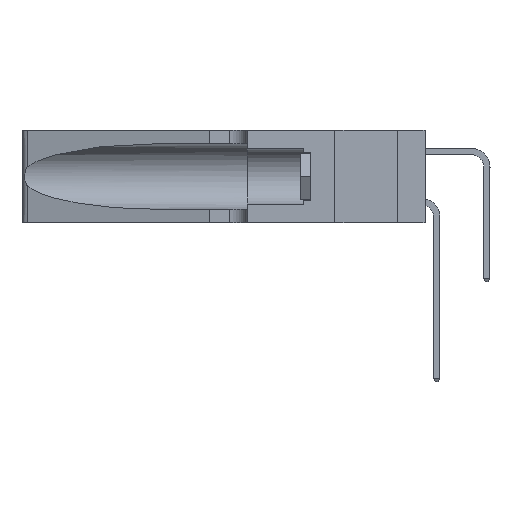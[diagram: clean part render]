
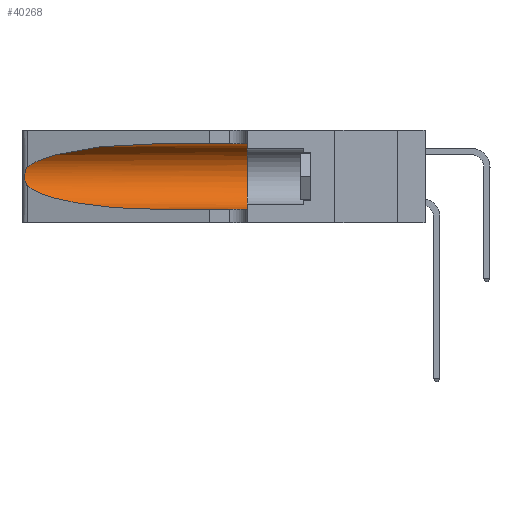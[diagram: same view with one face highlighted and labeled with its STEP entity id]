
A CAD part, left-side view. The second image highlights one B-rep face of the part: STEP entity #40268.
In plain terms, the highlighted cylindrical face has radius 3.308 mm (diameter 6.617 mm), a partial arc.
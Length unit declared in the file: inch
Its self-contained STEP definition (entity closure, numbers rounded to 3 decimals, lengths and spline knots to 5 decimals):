
#661 = B_SPLINE_CURVE_WITH_KNOTS ( 'NONE', 3,
 ( #7640, #23394, #4822, #4966, #5103, #8390, #40996, #11251, #28452, #34728, #28595, #31602, #32160, #907 ),
 .UNSPECIFIED., .F., .F.,
 ( 4, 2, 2, 2, 2, 2, 4 ),
 ( 0., 0.00027, 0.00053, 0.00107, 0.0016, 0.00187, 0.00214 ),
 .UNSPECIFIED. ) ;
#907 = CARTESIAN_POINT ( 'NONE',  ( 0.25487, 1.22718, 0.14631 ) ) ;
#982 = AXIS2_PLACEMENT_3D ( 'NONE', #37125, #40444, #34043 ) ;
#1090 = CARTESIAN_POINT ( 'NONE',  ( 0.25487, 1.22718, 0.22369 ) ) ;
#1676 = CARTESIAN_POINT ( 'NONE',  ( 0.18966, 0.96281, 0.05475 ) ) ;
#1841 = CARTESIAN_POINT ( 'NONE',  ( 0.1305, 1.61858, 0.05475 ) ) ;
#3299 = FACE_OUTER_BOUND ( 'NONE', #30682, .T. ) ;
#3983 = ORIENTED_EDGE ( 'NONE', *, *, #23581, .T. ) ;
#4087 = CARTESIAN_POINT ( 'NONE',  ( 0.1305, 0.35, 0.31525 ) ) ;
#4822 = CARTESIAN_POINT ( 'NONE',  ( 0.25639, 1.23184, 0.21858 ) ) ;
#4966 = CARTESIAN_POINT ( 'NONE',  ( 0.25787, 1.23484, 0.2124 ) ) ;
#5041 = CARTESIAN_POINT ( 'NONE',  ( 0.1305, 1.61858, 0.31525 ) ) ;
#5103 = CARTESIAN_POINT ( 'NONE',  ( 0.25854, 1.2359, 0.20912 ) ) ;
#6863 = DIRECTION ( 'NONE',  ( 0., 1., 0. ) ) ;
#6898 = CARTESIAN_POINT ( 'NONE',  ( 0.1305, 0.72297, 0.31525 ) ) ;
#7305 = CARTESIAN_POINT ( 'NONE',  ( 0.2373, 1.15595, 0.08982 ) ) ;
#7470 = CARTESIAN_POINT ( 'NONE',  ( 0.2373, 1.15595, 0.28018 ) ) ;
#7640 = CARTESIAN_POINT ( 'NONE',  ( 0.25487, 1.22718, 0.22369 ) ) ;
#7692 =( BOUNDED_CURVE ( )  B_SPLINE_CURVE ( 3, ( #14309, #7305, #1676, #37330 ),
 .UNSPECIFIED., .F., .F. ) 
 B_SPLINE_CURVE_WITH_KNOTS ( ( 4, 4 ),
 ( 3.44316, 4.71239 ),
 .UNSPECIFIED. ) 
 CURVE ( )  GEOMETRIC_REPRESENTATION_ITEM ( )  RATIONAL_B_SPLINE_CURVE ( ( 1., 0.87, 0.87, 1. ) ) 
 REPRESENTATION_ITEM ( '' )  );
#8259 =( BOUNDED_CURVE ( )  B_SPLINE_CURVE ( 3, ( #36243, #10764, #7470, #1090 ),
 .UNSPECIFIED., .F., .F. ) 
 B_SPLINE_CURVE_WITH_KNOTS ( ( 4, 4 ),
 ( 1.5708, 2.84003 ),
 .UNSPECIFIED. ) 
 CURVE ( )  GEOMETRIC_REPRESENTATION_ITEM ( )  RATIONAL_B_SPLINE_CURVE ( ( 1., 0.87, 0.87, 1. ) ) 
 REPRESENTATION_ITEM ( '' )  );
#8390 = CARTESIAN_POINT ( 'NONE',  ( 0.26018, 1.23835, 0.19895 ) ) ;
#10563 = VECTOR ( 'NONE', #34265, 39.37008 ) ;
#10764 = CARTESIAN_POINT ( 'NONE',  ( 0.18966, 0.96281, 0.31525 ) ) ;
#11251 = CARTESIAN_POINT ( 'NONE',  ( 0.26075, 1.23896, 0.178 ) ) ;
#13646 = VERTEX_POINT ( 'NONE', #27258 ) ;
#14309 = CARTESIAN_POINT ( 'NONE',  ( 0.25487, 1.22718, 0.14631 ) ) ;
#15715 = VERTEX_POINT ( 'NONE', #6898 ) ;
#16295 = CARTESIAN_POINT ( 'NONE',  ( 0.1305, 0.35, 0.185 ) ) ;
#17593 = VECTOR ( 'NONE', #31110, 39.37008 ) ;
#19251 = LINE ( 'NONE', #1841, #10563 ) ;
#19366 = EDGE_CURVE ( 'NONE', #25197, #13646, #7692, .T. ) ;
#20226 = ORIENTED_EDGE ( 'NONE', *, *, #36103, .F. ) ;
#20952 = EDGE_CURVE ( 'NONE', #13646, #32818, #19251, .T. ) ;
#23394 = CARTESIAN_POINT ( 'NONE',  ( 0.25555, 1.22994, 0.2215 ) ) ;
#23581 = EDGE_CURVE ( 'NONE', #15715, #36430, #8259, .T. ) ;
#24612 = AXIS2_PLACEMENT_3D ( 'NONE', #16295, #6863, #29396 ) ;
#24631 = CIRCLE ( 'NONE', #24612, 0.13025 ) ;
#24877 = EDGE_CURVE ( 'NONE', #36430, #25197, #661, .T. ) ;
#25197 = VERTEX_POINT ( 'NONE', #30613 ) ;
#27257 = LINE ( 'NONE', #5041, #17593 ) ;
#27258 = CARTESIAN_POINT ( 'NONE',  ( 0.1305, 0.72297, 0.05475 ) ) ;
#28452 = CARTESIAN_POINT ( 'NONE',  ( 0.26017, 1.23833, 0.17102 ) ) ;
#28595 = CARTESIAN_POINT ( 'NONE',  ( 0.25789, 1.23486, 0.15765 ) ) ;
#29396 = DIRECTION ( 'NONE',  ( 0., 0., 1. ) ) ;
#30114 = CARTESIAN_POINT ( 'NONE',  ( 0.1305, 0.35, 0.05475 ) ) ;
#30613 = CARTESIAN_POINT ( 'NONE',  ( 0.25487, 1.22718, 0.14631 ) ) ;
#30635 = ORIENTED_EDGE ( 'NONE', *, *, #20952, .T. ) ;
#30682 = EDGE_LOOP ( 'NONE', ( #3983, #35489, #35271, #30635, #20226, #39280 ) ) ;
#31110 = DIRECTION ( 'NONE',  ( 0., -1., 0. ) ) ;
#31602 = CARTESIAN_POINT ( 'NONE',  ( 0.25639, 1.23186, 0.15144 ) ) ;
#32160 = CARTESIAN_POINT ( 'NONE',  ( 0.25555, 1.22993, 0.14849 ) ) ;
#32818 = VERTEX_POINT ( 'NONE', #30114 ) ;
#33256 = CYLINDRICAL_SURFACE ( 'NONE', #982, 0.13025 ) ;
#34043 = DIRECTION ( 'NONE',  ( 0., 0., -1. ) ) ;
#34070 = CARTESIAN_POINT ( 'NONE',  ( 0.25487, 1.22718, 0.22369 ) ) ;
#34265 = DIRECTION ( 'NONE',  ( 0., -1., 0. ) ) ;
#34728 = CARTESIAN_POINT ( 'NONE',  ( 0.25856, 1.23593, 0.16098 ) ) ;
#35271 = ORIENTED_EDGE ( 'NONE', *, *, #19366, .T. ) ;
#35489 = ORIENTED_EDGE ( 'NONE', *, *, #24877, .T. ) ;
#36103 = EDGE_CURVE ( 'NONE', #38306, #32818, #24631, .T. ) ;
#36243 = CARTESIAN_POINT ( 'NONE',  ( 0.1305, 0.72297, 0.31525 ) ) ;
#36430 = VERTEX_POINT ( 'NONE', #34070 ) ;
#37125 = CARTESIAN_POINT ( 'NONE',  ( 0.1305, 1.61858, 0.185 ) ) ;
#37330 = CARTESIAN_POINT ( 'NONE',  ( 0.1305, 0.72297, 0.05475 ) ) ;
#38306 = VERTEX_POINT ( 'NONE', #4087 ) ;
#39203 = EDGE_CURVE ( 'NONE', #15715, #38306, #27257, .T. ) ;
#39280 = ORIENTED_EDGE ( 'NONE', *, *, #39203, .F. ) ;
#40268 = ADVANCED_FACE ( 'NONE', ( #3299 ), #33256, .F. ) ;
#40444 = DIRECTION ( 'NONE',  ( 0., -1., 0. ) ) ;
#40996 = CARTESIAN_POINT ( 'NONE',  ( 0.26075, 1.23896, 0.19203 ) ) ;
